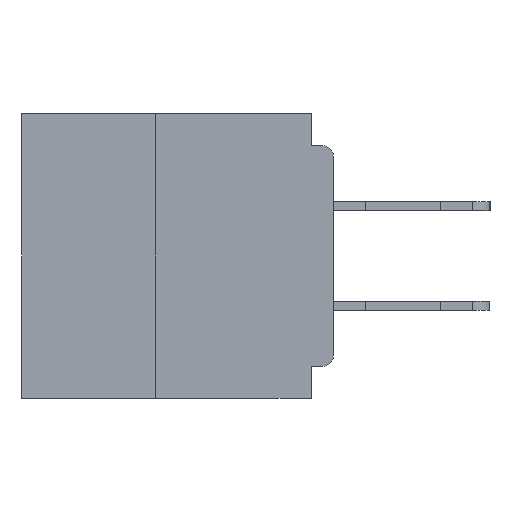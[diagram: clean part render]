
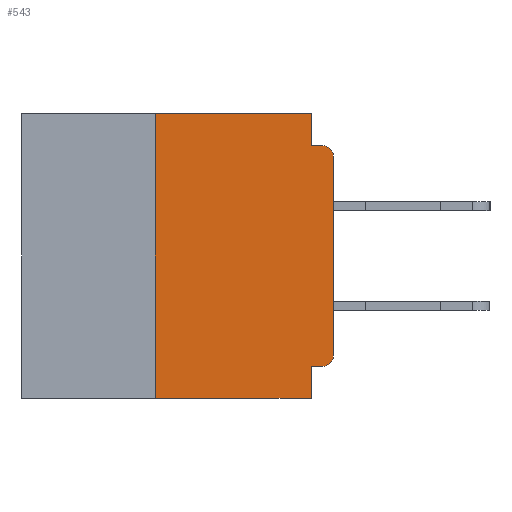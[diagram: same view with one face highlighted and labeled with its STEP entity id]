
A CAD part, left-side view. The second image highlights one B-rep face of the part: STEP entity #543.
In plain terms, the highlighted planar face has unit normal (-1, 0, 0).
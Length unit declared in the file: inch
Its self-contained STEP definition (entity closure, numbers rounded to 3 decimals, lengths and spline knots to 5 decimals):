
#2 = CARTESIAN_POINT ( 'NONE',  ( 0., 0., -0.045 ) ) ;
#543 = ADVANCED_FACE ( 'NONE', ( #677 ), #35047, .F. ) ;
#677 = FACE_OUTER_BOUND ( 'NONE', #17420, .T. ) ;
#1658 = CARTESIAN_POINT ( 'NONE',  ( 0., 0.031, 0. ) ) ;
#2099 = ORIENTED_EDGE ( 'NONE', *, *, #36181, .F. ) ;
#3618 = CIRCLE ( 'NONE', #37121, 0.015 ) ;
#4053 = CARTESIAN_POINT ( 'NONE',  ( 0., 0.25, 0. ) ) ;
#4203 = EDGE_CURVE ( 'NONE', #34389, #34290, #38994, .T. ) ;
#4336 = CARTESIAN_POINT ( 'NONE',  ( 0., 0.437, -0.4 ) ) ;
#4568 = EDGE_CURVE ( 'NONE', #13168, #16002, #23291, .T. ) ;
#4750 = LINE ( 'NONE', #37303, #22868 ) ;
#5233 = CARTESIAN_POINT ( 'NONE',  ( 0., 0.015, -0.34 ) ) ;
#5647 = VERTEX_POINT ( 'NONE', #49001 ) ;
#6170 = EDGE_CURVE ( 'NONE', #5647, #13168, #29133, .T. ) ;
#6770 = EDGE_CURVE ( 'NONE', #24094, #36868, #11513, .T. ) ;
#7012 = VERTEX_POINT ( 'NONE', #11176 ) ;
#7126 = ORIENTED_EDGE ( 'NONE', *, *, #12269, .F. ) ;
#7218 = DIRECTION ( 'NONE',  ( -1., 0., 0. ) ) ;
#8040 = CARTESIAN_POINT ( 'NONE',  ( 0., 0.437, 0. ) ) ;
#9095 = DIRECTION ( 'NONE',  ( 0., 0., -1. ) ) ;
#9668 = CARTESIAN_POINT ( 'NONE',  ( 0., 0., -0.06 ) ) ;
#10162 = ORIENTED_EDGE ( 'NONE', *, *, #6170, .T. ) ;
#11176 = CARTESIAN_POINT ( 'NONE',  ( 0., 0.031, -0.355 ) ) ;
#11513 = LINE ( 'NONE', #1658, #41095 ) ;
#12106 = DIRECTION ( 'NONE',  ( 0., 0., -1. ) ) ;
#12269 = EDGE_CURVE ( 'NONE', #15522, #7012, #15796, .T. ) ;
#13168 = VERTEX_POINT ( 'NONE', #9668 ) ;
#13818 = DIRECTION ( 'NONE',  ( 0., 0., 1. ) ) ;
#14593 = VECTOR ( 'NONE', #20563, 39.37008 ) ;
#14799 = VECTOR ( 'NONE', #19276, 39.37008 ) ;
#15522 = VERTEX_POINT ( 'NONE', #43797 ) ;
#15796 = LINE ( 'NONE', #39751, #14593 ) ;
#15867 = AXIS2_PLACEMENT_3D ( 'NONE', #30351, #7218, #34207 ) ;
#16002 = VERTEX_POINT ( 'NONE', #34904 ) ;
#17111 = ORIENTED_EDGE ( 'NONE', *, *, #6770, .F. ) ;
#17420 = EDGE_LOOP ( 'NONE', ( #10162, #28083, #47985, #17111, #32769, #49002, #46815, #2099, #7126, #36376 ) ) ;
#17584 = EDGE_CURVE ( 'NONE', #34290, #24094, #4750, .T. ) ;
#18300 = DIRECTION ( 'NONE',  ( 0., 0., 1. ) ) ;
#18888 = VECTOR ( 'NONE', #13818, 39.37008 ) ;
#19276 = DIRECTION ( 'NONE',  ( 0., -1., 0. ) ) ;
#19376 = CARTESIAN_POINT ( 'NONE',  ( 0., 0.031, -0.4 ) ) ;
#19699 = DIRECTION ( 'NONE',  ( 0., 0., -1. ) ) ;
#20563 = DIRECTION ( 'NONE',  ( 0., 1., 0. ) ) ;
#22868 = VECTOR ( 'NONE', #25491, 39.37008 ) ;
#23291 = CIRCLE ( 'NONE', #15867, 0.015 ) ;
#24094 = VERTEX_POINT ( 'NONE', #45404 ) ;
#24163 = AXIS2_PLACEMENT_3D ( 'NONE', #8040, #42726, #19699 ) ;
#25491 = DIRECTION ( 'NONE',  ( 0., -1., 0. ) ) ;
#27484 = CARTESIAN_POINT ( 'NONE',  ( 0., 0.031, -0.4 ) ) ;
#28083 = ORIENTED_EDGE ( 'NONE', *, *, #4568, .T. ) ;
#28782 = DIRECTION ( 'NONE',  ( 0., 0., -1. ) ) ;
#29133 = LINE ( 'NONE', #29185, #18888 ) ;
#29185 = CARTESIAN_POINT ( 'NONE',  ( 0., 0., 0. ) ) ;
#30351 = CARTESIAN_POINT ( 'NONE',  ( 0., 0.015, -0.06 ) ) ;
#31316 = DIRECTION ( 'NONE',  ( 0., -1., 0. ) ) ;
#31525 = CARTESIAN_POINT ( 'NONE',  ( 0., 0.25, -0.4 ) ) ;
#32232 = DIRECTION ( 'NONE',  ( -1., 0., 0. ) ) ;
#32769 = ORIENTED_EDGE ( 'NONE', *, *, #17584, .F. ) ;
#34207 = DIRECTION ( 'NONE',  ( 0., 0., -1. ) ) ;
#34290 = VERTEX_POINT ( 'NONE', #4053 ) ;
#34389 = VERTEX_POINT ( 'NONE', #31525 ) ;
#34904 = CARTESIAN_POINT ( 'NONE',  ( 0., 0.015, -0.045 ) ) ;
#35047 = PLANE ( 'NONE',  #24163 ) ;
#35321 = LINE ( 'NONE', #2, #14799 ) ;
#35531 = CARTESIAN_POINT ( 'NONE',  ( 0., 0.031, -0.045 ) ) ;
#35584 = EDGE_CURVE ( 'NONE', #36868, #16002, #35321, .T. ) ;
#35861 = VECTOR ( 'NONE', #12106, 39.37008 ) ;
#36181 = EDGE_CURVE ( 'NONE', #7012, #49150, #46004, .T. ) ;
#36376 = ORIENTED_EDGE ( 'NONE', *, *, #41662, .T. ) ;
#36868 = VERTEX_POINT ( 'NONE', #35531 ) ;
#37121 = AXIS2_PLACEMENT_3D ( 'NONE', #5233, #32232, #9095 ) ;
#37303 = CARTESIAN_POINT ( 'NONE',  ( 0., 0.437, 0. ) ) ;
#37808 = VECTOR ( 'NONE', #18300, 39.37008 ) ;
#38755 = EDGE_CURVE ( 'NONE', #34389, #49150, #44780, .T. ) ;
#38994 = LINE ( 'NONE', #45175, #37808 ) ;
#39751 = CARTESIAN_POINT ( 'NONE',  ( 0., 0., -0.355 ) ) ;
#41095 = VECTOR ( 'NONE', #28782, 39.37008 ) ;
#41662 = EDGE_CURVE ( 'NONE', #15522, #5647, #3618, .T. ) ;
#42726 = DIRECTION ( 'NONE',  ( 1., 0., 0. ) ) ;
#43596 = VECTOR ( 'NONE', #31316, 39.37008 ) ;
#43797 = CARTESIAN_POINT ( 'NONE',  ( 0., 0.015, -0.355 ) ) ;
#44780 = LINE ( 'NONE', #4336, #43596 ) ;
#45175 = CARTESIAN_POINT ( 'NONE',  ( 0., 0.25, -0.4 ) ) ;
#45404 = CARTESIAN_POINT ( 'NONE',  ( 0., 0.031, 0. ) ) ;
#46004 = LINE ( 'NONE', #27484, #35861 ) ;
#46815 = ORIENTED_EDGE ( 'NONE', *, *, #38755, .T. ) ;
#47985 = ORIENTED_EDGE ( 'NONE', *, *, #35584, .F. ) ;
#49001 = CARTESIAN_POINT ( 'NONE',  ( 0., 0., -0.34 ) ) ;
#49002 = ORIENTED_EDGE ( 'NONE', *, *, #4203, .F. ) ;
#49150 = VERTEX_POINT ( 'NONE', #19376 ) ;
